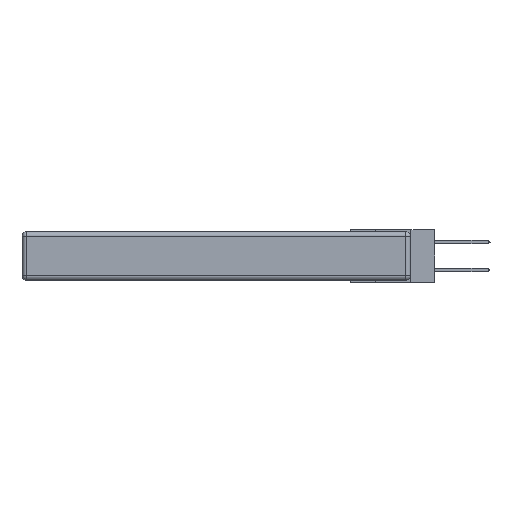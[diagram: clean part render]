
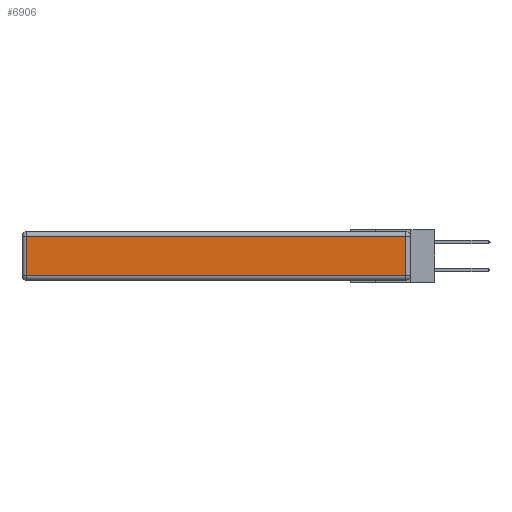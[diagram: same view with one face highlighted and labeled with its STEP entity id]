
A CAD part, left-side view. The second image highlights one B-rep face of the part: STEP entity #6906.
In plain terms, the highlighted planar face has unit normal (-1, 0, 0).
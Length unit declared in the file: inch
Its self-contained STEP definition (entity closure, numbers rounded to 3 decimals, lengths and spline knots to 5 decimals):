
#967 = VECTOR ( 'NONE', #11077, 39.37008 ) ;
#1102 = EDGE_LOOP ( 'NONE', ( #7503, #2749, #12636, #8756 ) ) ;
#1687 = CARTESIAN_POINT ( 'NONE',  ( 0., 0., -0.343 ) ) ;
#1927 = EDGE_CURVE ( 'NONE', #13181, #2735, #7065, .T. ) ;
#2049 = CARTESIAN_POINT ( 'NONE',  ( 0., 0., -0.313 ) ) ;
#2152 = FACE_OUTER_BOUND ( 'NONE', #1102, .T. ) ;
#2735 = VERTEX_POINT ( 'NONE', #3952 ) ;
#2749 = ORIENTED_EDGE ( 'NONE', *, *, #3073, .T. ) ;
#3073 = EDGE_CURVE ( 'NONE', #2735, #8494, #6955, .T. ) ;
#3431 = DIRECTION ( 'NONE',  ( 0., 0., -1. ) ) ;
#3774 = DIRECTION ( 'NONE',  ( 0., 0., 1. ) ) ;
#3919 = CARTESIAN_POINT ( 'NONE',  ( 0., 2.72, -0.313 ) ) ;
#3952 = CARTESIAN_POINT ( 'NONE',  ( 0., 0.03, -0.313 ) ) ;
#3966 = EDGE_CURVE ( 'NONE', #14824, #13181, #9425, .T. ) ;
#5144 = CARTESIAN_POINT ( 'NONE',  ( 0., 0.03, -0.03 ) ) ;
#6323 = CARTESIAN_POINT ( 'NONE',  ( 0., 2.72, -0.03 ) ) ;
#6538 = AXIS2_PLACEMENT_3D ( 'NONE', #1687, #7775, #3774 ) ;
#6906 = ADVANCED_FACE ( 'NONE', ( #2152 ), #11622, .T. ) ;
#6955 = LINE ( 'NONE', #9281, #12665 ) ;
#7065 = LINE ( 'NONE', #2049, #967 ) ;
#7503 = ORIENTED_EDGE ( 'NONE', *, *, #1927, .T. ) ;
#7556 = CARTESIAN_POINT ( 'NONE',  ( 0., 2.75, -0.03 ) ) ;
#7775 = DIRECTION ( 'NONE',  ( -1., 0., 0. ) ) ;
#8494 = VERTEX_POINT ( 'NONE', #5144 ) ;
#8658 = VECTOR ( 'NONE', #8746, 39.37008 ) ;
#8746 = DIRECTION ( 'NONE',  ( 0., 1., 0. ) ) ;
#8756 = ORIENTED_EDGE ( 'NONE', *, *, #3966, .T. ) ;
#9171 = LINE ( 'NONE', #7556, #8658 ) ;
#9281 = CARTESIAN_POINT ( 'NONE',  ( 0., 0.03, -0.343 ) ) ;
#9425 = LINE ( 'NONE', #12486, #10848 ) ;
#9868 = EDGE_CURVE ( 'NONE', #8494, #14824, #9171, .T. ) ;
#10848 = VECTOR ( 'NONE', #3431, 39.37008 ) ;
#11077 = DIRECTION ( 'NONE',  ( 0., -1., 0. ) ) ;
#11622 = PLANE ( 'NONE',  #6538 ) ;
#11674 = DIRECTION ( 'NONE',  ( 0., 0., 1. ) ) ;
#12486 = CARTESIAN_POINT ( 'NONE',  ( 0., 2.72, -0.343 ) ) ;
#12636 = ORIENTED_EDGE ( 'NONE', *, *, #9868, .T. ) ;
#12665 = VECTOR ( 'NONE', #11674, 39.37008 ) ;
#13181 = VERTEX_POINT ( 'NONE', #3919 ) ;
#14824 = VERTEX_POINT ( 'NONE', #6323 ) ;
